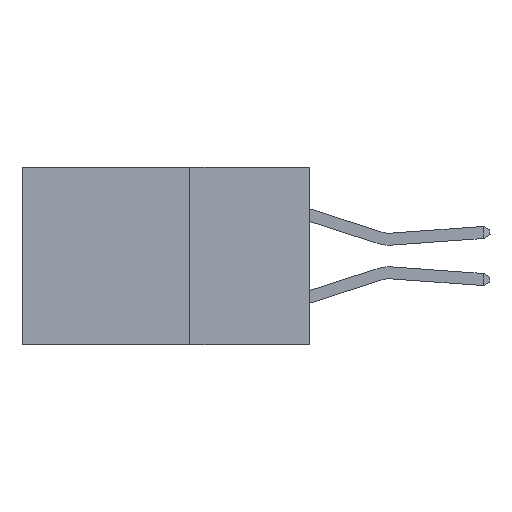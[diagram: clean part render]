
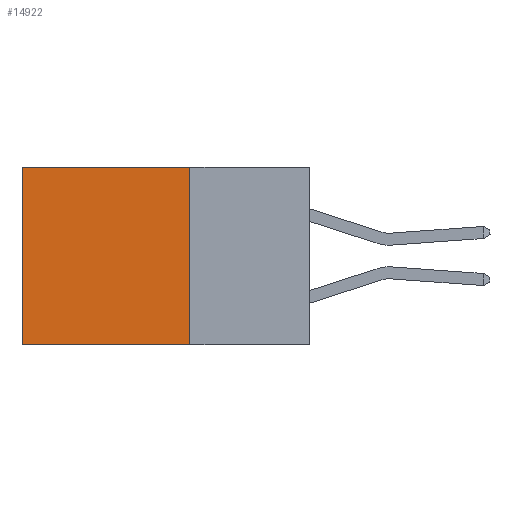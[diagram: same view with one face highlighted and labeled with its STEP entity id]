
A CAD part, left-side view. The second image highlights one B-rep face of the part: STEP entity #14922.
In plain terms, the highlighted planar face has unit normal (-1, 0, 0).
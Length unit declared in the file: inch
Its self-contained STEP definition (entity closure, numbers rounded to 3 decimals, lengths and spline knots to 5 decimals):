
#1420 = VERTEX_POINT ( 'NONE', #3165 ) ;
#2279 = VERTEX_POINT ( 'NONE', #6648 ) ;
#3165 = CARTESIAN_POINT ( 'NONE',  ( 0.298, 0.6, 0. ) ) ;
#3997 = CARTESIAN_POINT ( 'NONE',  ( 0.298, 0.25, 0. ) ) ;
#5516 = PLANE ( 'NONE',  #28201 ) ;
#6551 = EDGE_LOOP ( 'NONE', ( #21109, #19832, #7522, #18369 ) ) ;
#6648 = CARTESIAN_POINT ( 'NONE',  ( 0.298, 0.25, -0.37 ) ) ;
#7044 = LINE ( 'NONE', #10579, #21207 ) ;
#7149 = LINE ( 'NONE', #3997, #27183 ) ;
#7522 = ORIENTED_EDGE ( 'NONE', *, *, #19761, .F. ) ;
#8297 = EDGE_CURVE ( 'NONE', #13416, #1420, #7149, .T. ) ;
#8445 = DIRECTION ( 'NONE',  ( 0., 1., 0. ) ) ;
#9794 = EDGE_CURVE ( 'NONE', #2279, #25970, #7044, .T. ) ;
#10579 = CARTESIAN_POINT ( 'NONE',  ( 0.298, 0.25, -0.37 ) ) ;
#12220 = CARTESIAN_POINT ( 'NONE',  ( 0.298, 0.6, -0.37 ) ) ;
#13416 = VERTEX_POINT ( 'NONE', #17683 ) ;
#13643 = CARTESIAN_POINT ( 'NONE',  ( 0.298, 0.6, 0. ) ) ;
#14139 = DIRECTION ( 'NONE',  ( 0., 0., -1. ) ) ;
#14205 = FACE_OUTER_BOUND ( 'NONE', #6551, .T. ) ;
#14922 = ADVANCED_FACE ( 'NONE', ( #14205 ), #5516, .F. ) ;
#14951 = CARTESIAN_POINT ( 'NONE',  ( 0.298, 0.25, 0. ) ) ;
#15687 = DIRECTION ( 'NONE',  ( 0., 0., -1. ) ) ;
#16892 = LINE ( 'NONE', #13643, #23468 ) ;
#17683 = CARTESIAN_POINT ( 'NONE',  ( 0.298, 0.25, 0. ) ) ;
#18366 = DIRECTION ( 'NONE',  ( 1., 0., 0. ) ) ;
#18369 = ORIENTED_EDGE ( 'NONE', *, *, #8297, .T. ) ;
#19761 = EDGE_CURVE ( 'NONE', #13416, #2279, #28180, .T. ) ;
#19832 = ORIENTED_EDGE ( 'NONE', *, *, #9794, .F. ) ;
#21109 = ORIENTED_EDGE ( 'NONE', *, *, #23339, .T. ) ;
#21207 = VECTOR ( 'NONE', #8445, 39.37008 ) ;
#21893 = DIRECTION ( 'NONE',  ( 0., 1., 0. ) ) ;
#22336 = VECTOR ( 'NONE', #27249, 39.37008 ) ;
#23023 = CARTESIAN_POINT ( 'NONE',  ( 0.298, 0.25, 0. ) ) ;
#23339 = EDGE_CURVE ( 'NONE', #1420, #25970, #16892, .T. ) ;
#23468 = VECTOR ( 'NONE', #15687, 39.37008 ) ;
#25970 = VERTEX_POINT ( 'NONE', #12220 ) ;
#27183 = VECTOR ( 'NONE', #21893, 39.37008 ) ;
#27249 = DIRECTION ( 'NONE',  ( 0., 0., -1. ) ) ;
#28180 = LINE ( 'NONE', #14951, #22336 ) ;
#28201 = AXIS2_PLACEMENT_3D ( 'NONE', #23023, #18366, #14139 ) ;
